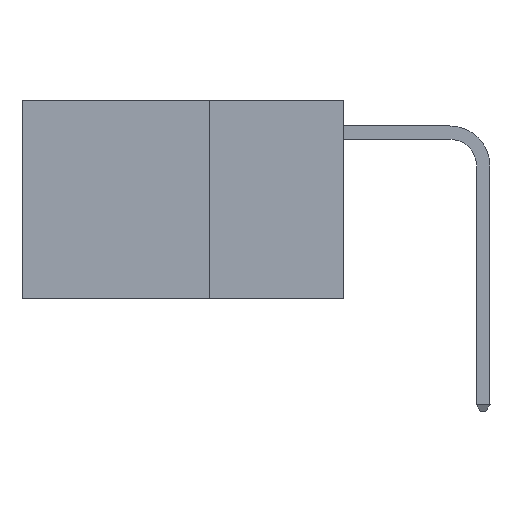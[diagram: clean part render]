
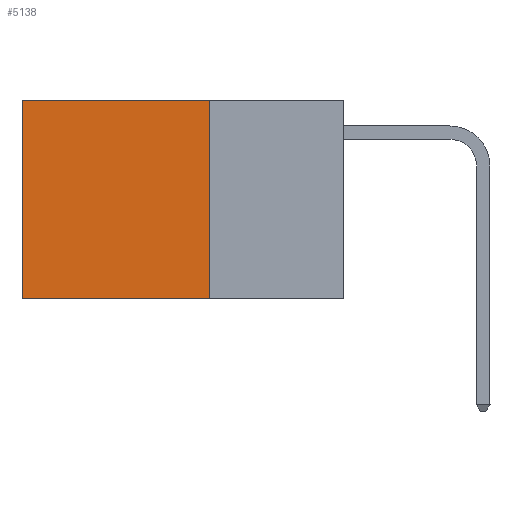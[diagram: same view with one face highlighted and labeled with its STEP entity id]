
A CAD part, left-side view. The second image highlights one B-rep face of the part: STEP entity #5138.
In plain terms, the highlighted planar face has unit normal (-1, 0, 0).
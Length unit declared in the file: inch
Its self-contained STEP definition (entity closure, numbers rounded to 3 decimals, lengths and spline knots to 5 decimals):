
#273 = DIRECTION ( 'NONE',  ( 1., 0., 0. ) ) ;
#531 = LINE ( 'NONE', #755, #8998 ) ;
#755 = CARTESIAN_POINT ( 'NONE',  ( 0.2625, 0.25, 0. ) ) ;
#1677 = EDGE_CURVE ( 'NONE', #16030, #18354, #11568, .T. ) ;
#1857 = ORIENTED_EDGE ( 'NONE', *, *, #14221, .F. ) ;
#4178 = ORIENTED_EDGE ( 'NONE', *, *, #20889, .T. ) ;
#5138 = ADVANCED_FACE ( 'NONE', ( #15827 ), #8719, .F. ) ;
#5341 = CARTESIAN_POINT ( 'NONE',  ( 0.2625, 0.6, 0. ) ) ;
#5436 = CARTESIAN_POINT ( 'NONE',  ( 0.2625, 0.25, 0. ) ) ;
#5955 = EDGE_CURVE ( 'NONE', #15571, #18354, #9112, .T. ) ;
#7094 = VECTOR ( 'NONE', #12785, 39.37008 ) ;
#7318 = ORIENTED_EDGE ( 'NONE', *, *, #1677, .T. ) ;
#7514 = CARTESIAN_POINT ( 'NONE',  ( 0.2625, 0.25, -0.37 ) ) ;
#8719 = PLANE ( 'NONE',  #18829 ) ;
#8998 = VECTOR ( 'NONE', #10882, 39.37008 ) ;
#9112 = LINE ( 'NONE', #12715, #12518 ) ;
#9522 = VERTEX_POINT ( 'NONE', #5436 ) ;
#9533 = EDGE_LOOP ( 'NONE', ( #7318, #14337, #1857, #4178 ) ) ;
#10882 = DIRECTION ( 'NONE',  ( 0., 0., -1. ) ) ;
#11051 = DIRECTION ( 'NONE',  ( 0., 1., 0. ) ) ;
#11568 = LINE ( 'NONE', #12758, #7094 ) ;
#11741 = CARTESIAN_POINT ( 'NONE',  ( 0.2625, 0.6, -0.37 ) ) ;
#12074 = DIRECTION ( 'NONE',  ( 0., 0., -1. ) ) ;
#12518 = VECTOR ( 'NONE', #11051, 39.37008 ) ;
#12715 = CARTESIAN_POINT ( 'NONE',  ( 0.2625, 0.25, -0.37 ) ) ;
#12758 = CARTESIAN_POINT ( 'NONE',  ( 0.2625, 0.6, 0. ) ) ;
#12785 = DIRECTION ( 'NONE',  ( 0., 0., -1. ) ) ;
#14221 = EDGE_CURVE ( 'NONE', #9522, #15571, #531, .T. ) ;
#14278 = DIRECTION ( 'NONE',  ( 0., 1., 0. ) ) ;
#14337 = ORIENTED_EDGE ( 'NONE', *, *, #5955, .F. ) ;
#15571 = VERTEX_POINT ( 'NONE', #7514 ) ;
#15827 = FACE_OUTER_BOUND ( 'NONE', #9533, .T. ) ;
#16030 = VERTEX_POINT ( 'NONE', #5341 ) ;
#16120 = VECTOR ( 'NONE', #14278, 39.37008 ) ;
#18354 = VERTEX_POINT ( 'NONE', #11741 ) ;
#18829 = AXIS2_PLACEMENT_3D ( 'NONE', #20202, #273, #12074 ) ;
#19054 = CARTESIAN_POINT ( 'NONE',  ( 0.2625, 0.25, 0. ) ) ;
#20202 = CARTESIAN_POINT ( 'NONE',  ( 0.2625, 0.25, 0. ) ) ;
#20388 = LINE ( 'NONE', #19054, #16120 ) ;
#20889 = EDGE_CURVE ( 'NONE', #9522, #16030, #20388, .T. ) ;
